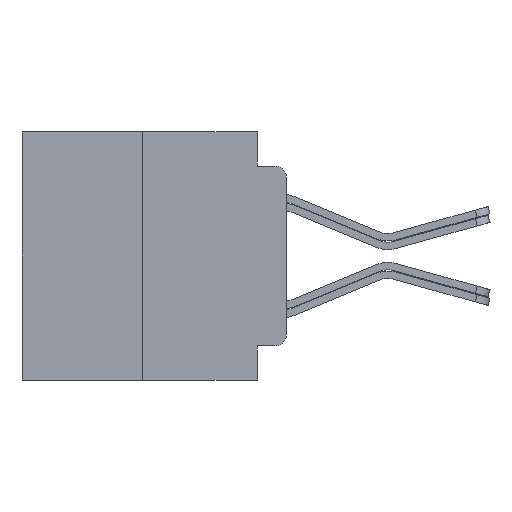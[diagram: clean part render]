
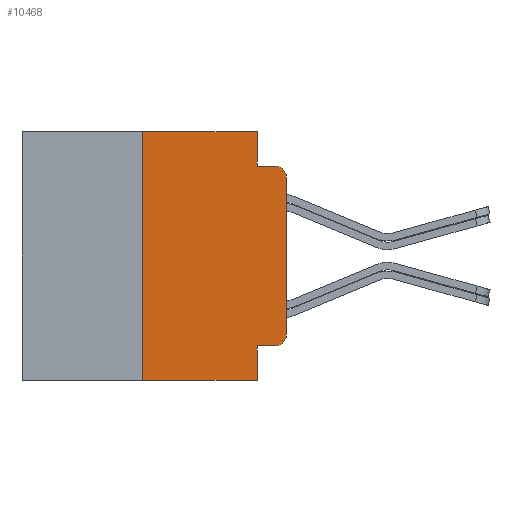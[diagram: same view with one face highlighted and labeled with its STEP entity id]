
A CAD part, left-side view. The second image highlights one B-rep face of the part: STEP entity #10468.
In plain terms, the highlighted planar face has unit normal (-1, 0, 0).
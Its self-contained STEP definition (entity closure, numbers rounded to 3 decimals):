
#609 = VECTOR ( 'NONE', #24020, 1000. ) ;
#775 = CARTESIAN_POINT ( 'NONE',  ( -75.603, 1.295, -5.486 ) ) ;
#801 = DIRECTION ( 'NONE',  ( -1., 0., 0. ) ) ;
#858 = EDGE_CURVE ( 'NONE', #3411, #16826, #19086, .T. ) ;
#904 = CARTESIAN_POINT ( 'NONE',  ( -75.603, 0., -3.467 ) ) ;
#950 = AXIS2_PLACEMENT_3D ( 'NONE', #11129, #801, #26955 ) ;
#1122 = DIRECTION ( 'NONE',  ( 0., -1., 0. ) ) ;
#1429 = VECTOR ( 'NONE', #4028, 1000. ) ;
#1579 = ORIENTED_EDGE ( 'NONE', *, *, #13099, .F. ) ;
#1640 = CARTESIAN_POINT ( 'NONE',  ( -75.603, 11.684, -5.486 ) ) ;
#1941 = CARTESIAN_POINT ( 'NONE',  ( -75.603, 6.35, -5.486 ) ) ;
#2353 = VERTEX_POINT ( 'NONE', #13473 ) ;
#2562 = VERTEX_POINT ( 'NONE', #18910 ) ;
#3411 = VERTEX_POINT ( 'NONE', #12634 ) ;
#3777 = ORIENTED_EDGE ( 'NONE', *, *, #23700, .T. ) ;
#3825 = CARTESIAN_POINT ( 'NONE',  ( -75.603, 1.295, 5.486 ) ) ;
#4028 = DIRECTION ( 'NONE',  ( 0., -1., 0. ) ) ;
#4042 = CARTESIAN_POINT ( 'NONE',  ( -75.603, 0., 3.467 ) ) ;
#4340 = VERTEX_POINT ( 'NONE', #10596 ) ;
#4540 = ORIENTED_EDGE ( 'NONE', *, *, #8090, .T. ) ;
#4876 = CARTESIAN_POINT ( 'NONE',  ( -75.603, 1.295, -3.975 ) ) ;
#5028 = LINE ( 'NONE', #23659, #19573 ) ;
#7152 = VERTEX_POINT ( 'NONE', #17080 ) ;
#7507 = CIRCLE ( 'NONE', #12789, 0.508 ) ;
#8090 = EDGE_CURVE ( 'NONE', #26205, #2562, #9826, .T. ) ;
#8590 = LINE ( 'NONE', #15598, #17243 ) ;
#9826 = CIRCLE ( 'NONE', #950, 0.508 ) ;
#10069 = VECTOR ( 'NONE', #1122, 1000. ) ;
#10215 = ORIENTED_EDGE ( 'NONE', *, *, #15344, .F. ) ;
#10468 = ADVANCED_FACE ( 'NONE', ( #19369 ), #10583, .F. ) ;
#10503 = EDGE_CURVE ( 'NONE', #7152, #23702, #22507, .T. ) ;
#10583 = PLANE ( 'NONE',  #13704 ) ;
#10596 = CARTESIAN_POINT ( 'NONE',  ( -75.603, 6.35, 5.486 ) ) ;
#10760 = LINE ( 'NONE', #23375, #10069 ) ;
#10812 = VECTOR ( 'NONE', #23197, 1000. ) ;
#11129 = CARTESIAN_POINT ( 'NONE',  ( -75.603, 0.508, 3.467 ) ) ;
#11234 = DIRECTION ( 'NONE',  ( 0., 0., 1. ) ) ;
#11946 = EDGE_CURVE ( 'NONE', #3411, #4340, #17530, .T. ) ;
#12456 = VERTEX_POINT ( 'NONE', #3825 ) ;
#12634 = CARTESIAN_POINT ( 'NONE',  ( -75.603, 6.35, -5.486 ) ) ;
#12781 = CARTESIAN_POINT ( 'NONE',  ( -75.603, 0.508, -3.467 ) ) ;
#12789 = AXIS2_PLACEMENT_3D ( 'NONE', #12781, #23755, #28321 ) ;
#13048 = DIRECTION ( 'NONE',  ( 0., 0., -1. ) ) ;
#13086 = CARTESIAN_POINT ( 'NONE',  ( -75.603, 11.684, 5.486 ) ) ;
#13099 = EDGE_CURVE ( 'NONE', #2353, #2562, #5028, .T. ) ;
#13368 = ORIENTED_EDGE ( 'NONE', *, *, #16328, .F. ) ;
#13473 = CARTESIAN_POINT ( 'NONE',  ( -75.603, 1.295, 3.975 ) ) ;
#13704 = AXIS2_PLACEMENT_3D ( 'NONE', #13086, #19597, #26128 ) ;
#14079 = CARTESIAN_POINT ( 'NONE',  ( -75.603, 1.295, 0. ) ) ;
#15344 = EDGE_CURVE ( 'NONE', #12456, #2353, #20146, .T. ) ;
#15598 = CARTESIAN_POINT ( 'NONE',  ( -75.603, 0., 5.486 ) ) ;
#15630 = DIRECTION ( 'NONE',  ( 0., -1., 0. ) ) ;
#16328 = EDGE_CURVE ( 'NONE', #4340, #12456, #10760, .T. ) ;
#16826 = VERTEX_POINT ( 'NONE', #775 ) ;
#17080 = CARTESIAN_POINT ( 'NONE',  ( -75.603, 1.295, -3.975 ) ) ;
#17243 = VECTOR ( 'NONE', #11234, 1000. ) ;
#17439 = ORIENTED_EDGE ( 'NONE', *, *, #10503, .T. ) ;
#17530 = LINE ( 'NONE', #1941, #609 ) ;
#18910 = CARTESIAN_POINT ( 'NONE',  ( -75.603, 0.508, 3.975 ) ) ;
#19086 = LINE ( 'NONE', #1640, #1429 ) ;
#19105 = DIRECTION ( 'NONE',  ( 0., -1., 0. ) ) ;
#19369 = FACE_OUTER_BOUND ( 'NONE', #27185, .T. ) ;
#19488 = CARTESIAN_POINT ( 'NONE',  ( -75.603, 0.508, -3.975 ) ) ;
#19573 = VECTOR ( 'NONE', #19105, 1000. ) ;
#19597 = DIRECTION ( 'NONE',  ( 1., 0., 0. ) ) ;
#20146 = LINE ( 'NONE', #26378, #22934 ) ;
#20587 = ORIENTED_EDGE ( 'NONE', *, *, #11946, .F. ) ;
#20889 = ORIENTED_EDGE ( 'NONE', *, *, #28457, .F. ) ;
#22312 = EDGE_CURVE ( 'NONE', #24246, #26205, #8590, .T. ) ;
#22507 = LINE ( 'NONE', #4876, #27729 ) ;
#22934 = VECTOR ( 'NONE', #13048, 1000. ) ;
#23197 = DIRECTION ( 'NONE',  ( 0., 0., -1. ) ) ;
#23375 = CARTESIAN_POINT ( 'NONE',  ( -75.603, 11.684, 5.486 ) ) ;
#23659 = CARTESIAN_POINT ( 'NONE',  ( -75.603, 1.295, 3.975 ) ) ;
#23700 = EDGE_CURVE ( 'NONE', #23702, #24246, #7507, .T. ) ;
#23702 = VERTEX_POINT ( 'NONE', #19488 ) ;
#23755 = DIRECTION ( 'NONE',  ( -1., 0., 0. ) ) ;
#24020 = DIRECTION ( 'NONE',  ( 0., 0., 1. ) ) ;
#24246 = VERTEX_POINT ( 'NONE', #904 ) ;
#26128 = DIRECTION ( 'NONE',  ( 0., 0., -1. ) ) ;
#26205 = VERTEX_POINT ( 'NONE', #4042 ) ;
#26241 = ORIENTED_EDGE ( 'NONE', *, *, #22312, .T. ) ;
#26378 = CARTESIAN_POINT ( 'NONE',  ( -75.603, 1.295, 0. ) ) ;
#26792 = LINE ( 'NONE', #14079, #10812 ) ;
#26955 = DIRECTION ( 'NONE',  ( 0., 0., -1. ) ) ;
#27132 = ORIENTED_EDGE ( 'NONE', *, *, #858, .T. ) ;
#27185 = EDGE_LOOP ( 'NONE', ( #17439, #3777, #26241, #4540, #1579, #10215, #13368, #20587, #27132, #20889 ) ) ;
#27729 = VECTOR ( 'NONE', #15630, 1000. ) ;
#28321 = DIRECTION ( 'NONE',  ( 0., 0., -1. ) ) ;
#28457 = EDGE_CURVE ( 'NONE', #7152, #16826, #26792, .T. ) ;
